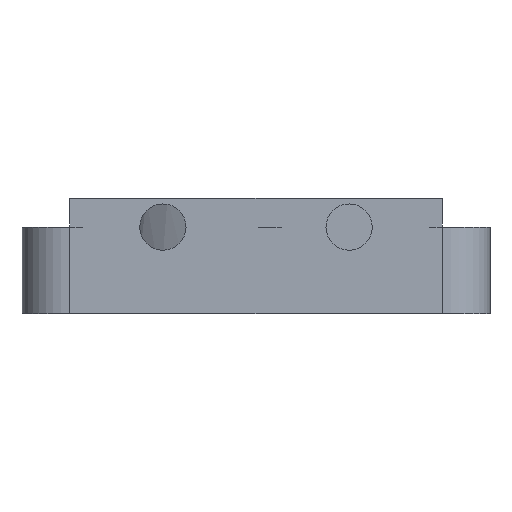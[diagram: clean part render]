
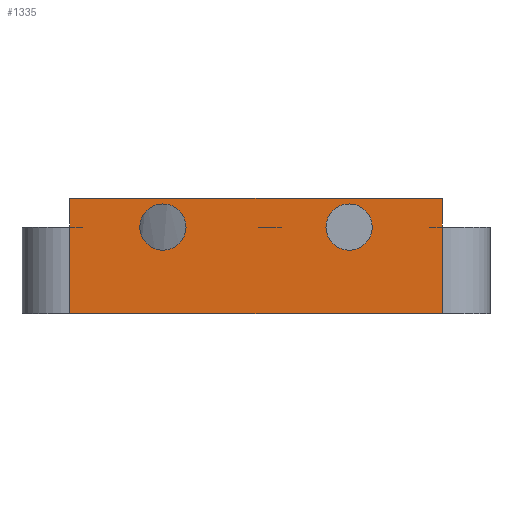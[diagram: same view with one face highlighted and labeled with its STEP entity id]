
A CAD part, front view. The second image highlights one B-rep face of the part: STEP entity #1335.
In plain terms, the highlighted planar face has unit normal (0, -1, 0).
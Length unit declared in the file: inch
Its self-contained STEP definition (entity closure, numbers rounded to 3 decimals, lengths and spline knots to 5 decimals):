
#41 = ORIENTED_EDGE ( 'NONE', *, *, #331, .T. ) ;
#48 = CIRCLE ( 'NONE', #121, 0.8 ) ;
#85 = LINE ( 'NONE', #494, #1264 ) ;
#91 = VERTEX_POINT ( 'NONE', #1395 ) ;
#105 = AXIS2_PLACEMENT_3D ( 'NONE', #779, #559, #435 ) ;
#121 = AXIS2_PLACEMENT_3D ( 'NONE', #572, #563, #555 ) ;
#124 = VERTEX_POINT ( 'NONE', #1168 ) ;
#159 = CARTESIAN_POINT ( 'NONE',  ( 13.25883, 3.5099, 3.8 ) ) ;
#179 = LINE ( 'NONE', #1330, #810 ) ;
#204 = EDGE_CURVE ( 'NONE', #616, #91, #401, .T. ) ;
#231 = EDGE_CURVE ( 'NONE', #455, #872, #48, .T. ) ;
#240 = VERTEX_POINT ( 'NONE', #579 ) ;
#248 = EDGE_CURVE ( 'NONE', #616, #712, #670, .T. ) ;
#275 = DIRECTION ( 'NONE',  ( 0., 0., -1. ) ) ;
#331 = EDGE_CURVE ( 'NONE', #124, #698, #1463, .T. ) ;
#400 = CARTESIAN_POINT ( 'NONE',  ( 16.47817, 3.5099, 4. ) ) ;
#401 = LINE ( 'NONE', #904, #1030 ) ;
#414 = ORIENTED_EDGE ( 'NONE', *, *, #231, .T. ) ;
#425 = LINE ( 'NONE', #1388, #699 ) ;
#433 = EDGE_CURVE ( 'NONE', #712, #240, #85, .T. ) ;
#435 = DIRECTION ( 'NONE',  ( 1., 0., 0. ) ) ;
#445 = CARTESIAN_POINT ( 'NONE',  ( 16.47817, 3.5099, 4. ) ) ;
#447 = DIRECTION ( 'NONE',  ( -1., 0., 0. ) ) ;
#453 = FACE_BOUND ( 'NONE', #1218, .T. ) ;
#455 = VERTEX_POINT ( 'NONE', #159 ) ;
#465 = DIRECTION ( 'NONE',  ( 0., 0., -1. ) ) ;
#494 = CARTESIAN_POINT ( 'NONE',  ( 16.47817, 3.5099, 4. ) ) ;
#512 = CARTESIAN_POINT ( 'NONE',  ( 16.47817, 3.5099, 3. ) ) ;
#513 = EDGE_CURVE ( 'NONE', #872, #455, #885, .T. ) ;
#555 = DIRECTION ( 'NONE',  ( 1., 0., 0. ) ) ;
#559 = DIRECTION ( 'NONE',  ( 0., 1., 0. ) ) ;
#563 = DIRECTION ( 'NONE',  ( 0., 1., 0. ) ) ;
#565 = EDGE_LOOP ( 'NONE', ( #1258, #1328, #1132, #1094, #1357, #1042 ) ) ;
#572 = CARTESIAN_POINT ( 'NONE',  ( 13.25883, 3.5099, 3. ) ) ;
#579 = CARTESIAN_POINT ( 'NONE',  ( 16.47817, 3.5099, 0. ) ) ;
#608 = CARTESIAN_POINT ( 'NONE',  ( 3.60082, 3.5099, 4. ) ) ;
#616 = VERTEX_POINT ( 'NONE', #400 ) ;
#670 = LINE ( 'NONE', #445, #1525 ) ;
#698 = VERTEX_POINT ( 'NONE', #746 ) ;
#699 = VECTOR ( 'NONE', #447, 39.37008 ) ;
#712 = VERTEX_POINT ( 'NONE', #512 ) ;
#746 = CARTESIAN_POINT ( 'NONE',  ( 6.82016, 3.5099, 2.2 ) ) ;
#766 = AXIS2_PLACEMENT_3D ( 'NONE', #980, #973, #1429 ) ;
#773 = FACE_BOUND ( 'NONE', #910, .T. ) ;
#779 = CARTESIAN_POINT ( 'NONE',  ( 6.82016, 3.5099, 3. ) ) ;
#810 = VECTOR ( 'NONE', #862, 39.37008 ) ;
#862 = DIRECTION ( 'NONE',  ( 0., 0., -1. ) ) ;
#868 = DIRECTION ( 'NONE',  ( 0., 0., -1. ) ) ;
#872 = VERTEX_POINT ( 'NONE', #1484 ) ;
#885 = CIRCLE ( 'NONE', #1378, 0.8 ) ;
#886 = AXIS2_PLACEMENT_3D ( 'NONE', #1412, #1326, #1318 ) ;
#904 = CARTESIAN_POINT ( 'NONE',  ( 0., 3.5099, 4. ) ) ;
#910 = EDGE_LOOP ( 'NONE', ( #1456, #41 ) ) ;
#922 = DIRECTION ( 'NONE',  ( -1., 0., 0. ) ) ;
#973 = DIRECTION ( 'NONE',  ( 0., -1., 0. ) ) ;
#980 = CARTESIAN_POINT ( 'NONE',  ( 0., 3.5099, 4. ) ) ;
#1013 = EDGE_CURVE ( 'NONE', #1135, #1069, #179, .T. ) ;
#1030 = VECTOR ( 'NONE', #922, 39.37008 ) ;
#1042 = ORIENTED_EDGE ( 'NONE', *, *, #1013, .T. ) ;
#1069 = VERTEX_POINT ( 'NONE', #1300 ) ;
#1094 = ORIENTED_EDGE ( 'NONE', *, *, #204, .T. ) ;
#1130 = VECTOR ( 'NONE', #868, 39.37008 ) ;
#1132 = ORIENTED_EDGE ( 'NONE', *, *, #248, .F. ) ;
#1135 = VERTEX_POINT ( 'NONE', #1297 ) ;
#1168 = CARTESIAN_POINT ( 'NONE',  ( 6.82016, 3.5099, 3.8 ) ) ;
#1190 = LINE ( 'NONE', #608, #1130 ) ;
#1218 = EDGE_LOOP ( 'NONE', ( #1411, #414 ) ) ;
#1223 = CIRCLE ( 'NONE', #105, 0.8 ) ;
#1258 = ORIENTED_EDGE ( 'NONE', *, *, #1457, .F. ) ;
#1264 = VECTOR ( 'NONE', #275, 39.37008 ) ;
#1281 = EDGE_CURVE ( 'NONE', #91, #1135, #1190, .T. ) ;
#1297 = CARTESIAN_POINT ( 'NONE',  ( 3.60082, 3.5099, 3. ) ) ;
#1300 = CARTESIAN_POINT ( 'NONE',  ( 3.60082, 3.5099, 0. ) ) ;
#1318 = DIRECTION ( 'NONE',  ( 1., 0., 0. ) ) ;
#1326 = DIRECTION ( 'NONE',  ( 0., 1., 0. ) ) ;
#1328 = ORIENTED_EDGE ( 'NONE', *, *, #433, .F. ) ;
#1330 = CARTESIAN_POINT ( 'NONE',  ( 3.60082, 3.5099, 4. ) ) ;
#1335 = ADVANCED_FACE ( 'NONE', ( #773, #1392, #453 ), #1338, .T. ) ;
#1338 = PLANE ( 'NONE',  #766 ) ;
#1340 = DIRECTION ( 'NONE',  ( 1., 0., 0. ) ) ;
#1357 = ORIENTED_EDGE ( 'NONE', *, *, #1281, .T. ) ;
#1378 = AXIS2_PLACEMENT_3D ( 'NONE', #1443, #1434, #1340 ) ;
#1388 = CARTESIAN_POINT ( 'NONE',  ( 0., 3.5099, 0. ) ) ;
#1392 = FACE_OUTER_BOUND ( 'NONE', #565, .T. ) ;
#1395 = CARTESIAN_POINT ( 'NONE',  ( 3.60082, 3.5099, 4. ) ) ;
#1411 = ORIENTED_EDGE ( 'NONE', *, *, #513, .T. ) ;
#1412 = CARTESIAN_POINT ( 'NONE',  ( 6.82016, 3.5099, 3. ) ) ;
#1429 = DIRECTION ( 'NONE',  ( 1., 0., 0. ) ) ;
#1434 = DIRECTION ( 'NONE',  ( 0., 1., 0. ) ) ;
#1443 = CARTESIAN_POINT ( 'NONE',  ( 13.25883, 3.5099, 3. ) ) ;
#1456 = ORIENTED_EDGE ( 'NONE', *, *, #1512, .T. ) ;
#1457 = EDGE_CURVE ( 'NONE', #240, #1069, #425, .T. ) ;
#1463 = CIRCLE ( 'NONE', #886, 0.8 ) ;
#1484 = CARTESIAN_POINT ( 'NONE',  ( 13.25883, 3.5099, 2.2 ) ) ;
#1512 = EDGE_CURVE ( 'NONE', #698, #124, #1223, .T. ) ;
#1525 = VECTOR ( 'NONE', #465, 39.37008 ) ;
